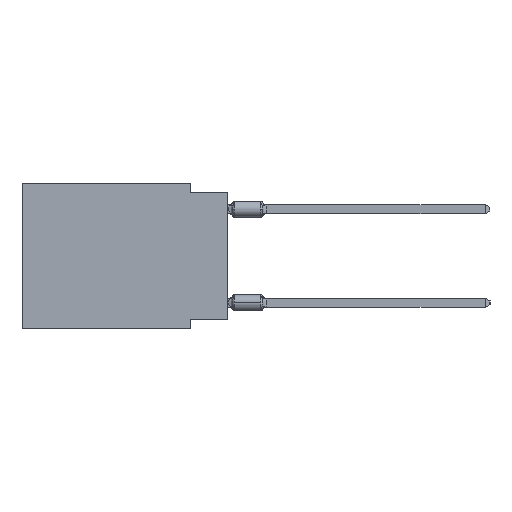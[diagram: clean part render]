
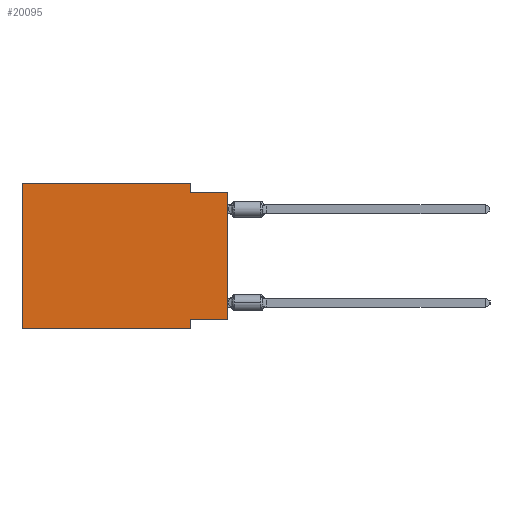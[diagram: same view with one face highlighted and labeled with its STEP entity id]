
A CAD part, left-side view. The second image highlights one B-rep face of the part: STEP entity #20095.
In plain terms, the highlighted planar face has unit normal (-1, 0, 0).
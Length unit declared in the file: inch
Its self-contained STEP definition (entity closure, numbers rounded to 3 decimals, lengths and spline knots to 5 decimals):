
#188 = CARTESIAN_POINT ( 'NONE',  ( 0., 0.55, -0.39 ) ) ;
#2367 = LINE ( 'NONE', #16335, #38333 ) ;
#3156 = VECTOR ( 'NONE', #32687, 39.37008 ) ;
#3178 = CARTESIAN_POINT ( 'NONE',  ( 0., 0.1, 0. ) ) ;
#3732 = LINE ( 'NONE', #188, #15424 ) ;
#5360 = VERTEX_POINT ( 'NONE', #17530 ) ;
#7569 = ORIENTED_EDGE ( 'NONE', *, *, #9392, .F. ) ;
#7946 = EDGE_CURVE ( 'NONE', #19980, #8687, #3732, .T. ) ;
#8614 = VECTOR ( 'NONE', #33098, 39.37008 ) ;
#8687 = VERTEX_POINT ( 'NONE', #14262 ) ;
#8725 = VERTEX_POINT ( 'NONE', #28164 ) ;
#8934 = DIRECTION ( 'NONE',  ( 0., 0., 1. ) ) ;
#9392 = EDGE_CURVE ( 'NONE', #31759, #8687, #45195, .T. ) ;
#9730 = DIRECTION ( 'NONE',  ( 0., 0., 1. ) ) ;
#10858 = CARTESIAN_POINT ( 'NONE',  ( 0., 0.55, -0.39 ) ) ;
#11801 = DIRECTION ( 'NONE',  ( 0., 0., -1. ) ) ;
#13048 = CARTESIAN_POINT ( 'NONE',  ( 0., 0., 0. ) ) ;
#14262 = CARTESIAN_POINT ( 'NONE',  ( 0., 0.1, -0.39 ) ) ;
#14521 = CARTESIAN_POINT ( 'NONE',  ( 0., 0.1, -0.025 ) ) ;
#14662 = AXIS2_PLACEMENT_3D ( 'NONE', #44056, #40062, #11801 ) ;
#14977 = EDGE_CURVE ( 'NONE', #8725, #38420, #18549, .T. ) ;
#15218 = EDGE_CURVE ( 'NONE', #41080, #31759, #15479, .T. ) ;
#15424 = VECTOR ( 'NONE', #35127, 39.37008 ) ;
#15479 = LINE ( 'NONE', #26072, #41156 ) ;
#16335 = CARTESIAN_POINT ( 'NONE',  ( 0., 0.55, 0. ) ) ;
#16827 = LINE ( 'NONE', #13048, #23400 ) ;
#17530 = CARTESIAN_POINT ( 'NONE',  ( 0., 0.55, 0. ) ) ;
#18549 = LINE ( 'NONE', #3178, #3156 ) ;
#18626 = ORIENTED_EDGE ( 'NONE', *, *, #15218, .F. ) ;
#18748 = ORIENTED_EDGE ( 'NONE', *, *, #45034, .T. ) ;
#19980 = VERTEX_POINT ( 'NONE', #10858 ) ;
#20019 = CARTESIAN_POINT ( 'NONE',  ( 0., 0.1, -0.39 ) ) ;
#20095 = ADVANCED_FACE ( 'NONE', ( #40302 ), #33480, .F. ) ;
#20235 = DIRECTION ( 'NONE',  ( 0., 0., -1. ) ) ;
#22884 = CARTESIAN_POINT ( 'NONE',  ( 0., 0.55, 0. ) ) ;
#23400 = VECTOR ( 'NONE', #9730, 39.37008 ) ;
#23459 = VECTOR ( 'NONE', #8934, 39.37008 ) ;
#24099 = ORIENTED_EDGE ( 'NONE', *, *, #7946, .T. ) ;
#24661 = ORIENTED_EDGE ( 'NONE', *, *, #41636, .F. ) ;
#25244 = VECTOR ( 'NONE', #20235, 39.37008 ) ;
#26072 = CARTESIAN_POINT ( 'NONE',  ( 0., 0., -0.365 ) ) ;
#26529 = DIRECTION ( 'NONE',  ( 0., 1., 0. ) ) ;
#27341 = LINE ( 'NONE', #22884, #23459 ) ;
#27705 = ORIENTED_EDGE ( 'NONE', *, *, #28056, .F. ) ;
#28056 = EDGE_CURVE ( 'NONE', #5360, #8725, #2367, .T. ) ;
#28164 = CARTESIAN_POINT ( 'NONE',  ( 0., 0.1, 0. ) ) ;
#29314 = ORIENTED_EDGE ( 'NONE', *, *, #36554, .F. ) ;
#31759 = VERTEX_POINT ( 'NONE', #41015 ) ;
#32687 = DIRECTION ( 'NONE',  ( 0., 0., -1. ) ) ;
#33098 = DIRECTION ( 'NONE',  ( 0., -1., 0. ) ) ;
#33480 = PLANE ( 'NONE',  #14662 ) ;
#34477 = DIRECTION ( 'NONE',  ( 0., -1., 0. ) ) ;
#35127 = DIRECTION ( 'NONE',  ( 0., -1., 0. ) ) ;
#36554 = EDGE_CURVE ( 'NONE', #19980, #5360, #27341, .T. ) ;
#38333 = VECTOR ( 'NONE', #34477, 39.37008 ) ;
#38420 = VERTEX_POINT ( 'NONE', #14521 ) ;
#39241 = CARTESIAN_POINT ( 'NONE',  ( 0., 0., -0.365 ) ) ;
#39911 = LINE ( 'NONE', #40616, #8614 ) ;
#40062 = DIRECTION ( 'NONE',  ( 1., 0., 0. ) ) ;
#40302 = FACE_OUTER_BOUND ( 'NONE', #44041, .T. ) ;
#40616 = CARTESIAN_POINT ( 'NONE',  ( 0., 0., -0.025 ) ) ;
#41015 = CARTESIAN_POINT ( 'NONE',  ( 0., 0.1, -0.365 ) ) ;
#41051 = CARTESIAN_POINT ( 'NONE',  ( 0., 0., -0.025 ) ) ;
#41080 = VERTEX_POINT ( 'NONE', #39241 ) ;
#41156 = VECTOR ( 'NONE', #26529, 39.37008 ) ;
#41636 = EDGE_CURVE ( 'NONE', #38420, #46516, #39911, .T. ) ;
#44041 = EDGE_LOOP ( 'NONE', ( #18748, #24661, #45900, #27705, #29314, #24099, #7569, #18626 ) ) ;
#44056 = CARTESIAN_POINT ( 'NONE',  ( 0., 0.55, 0. ) ) ;
#45034 = EDGE_CURVE ( 'NONE', #41080, #46516, #16827, .T. ) ;
#45195 = LINE ( 'NONE', #20019, #25244 ) ;
#45900 = ORIENTED_EDGE ( 'NONE', *, *, #14977, .F. ) ;
#46516 = VERTEX_POINT ( 'NONE', #41051 ) ;
